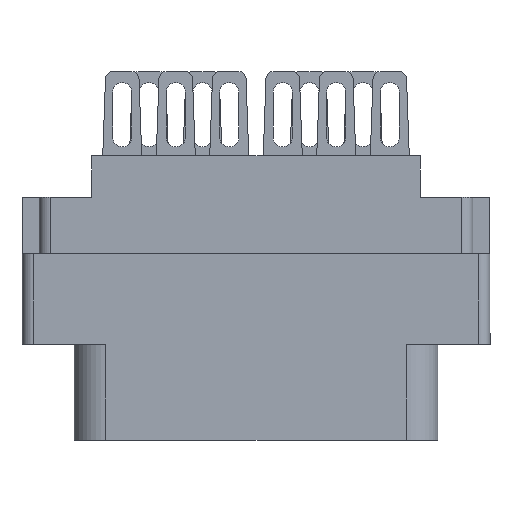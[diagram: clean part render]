
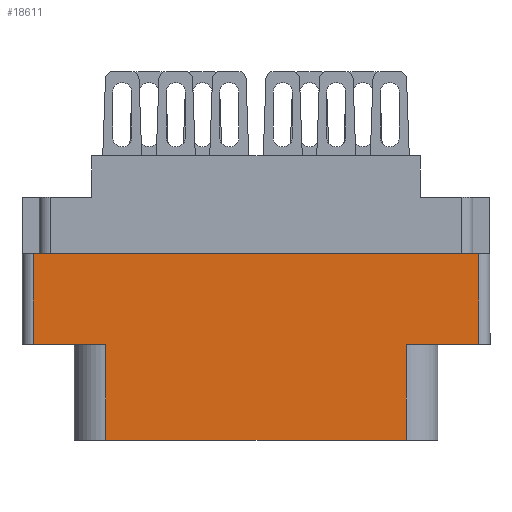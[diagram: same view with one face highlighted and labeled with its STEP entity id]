
A CAD part, front view. The second image highlights one B-rep face of the part: STEP entity #18611.
In plain terms, the highlighted planar face has unit normal (0, -1, 0).
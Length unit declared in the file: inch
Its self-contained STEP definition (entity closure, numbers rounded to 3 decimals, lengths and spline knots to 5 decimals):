
#87 = DIRECTION ( 'NONE',  ( 0., 0., 1. ) ) ;
#232 = VERTEX_POINT ( 'NONE', #1029 ) ;
#833 = LINE ( 'NONE', #1506, #4343 ) ;
#1029 = CARTESIAN_POINT ( 'NONE',  ( -0.42052, -0.343, -0.798 ) ) ;
#1467 = ORIENTED_EDGE ( 'NONE', *, *, #18213, .T. ) ;
#1506 = CARTESIAN_POINT ( 'NONE',  ( -0.624, -0.343, -0.798 ) ) ;
#1854 = ORIENTED_EDGE ( 'NONE', *, *, #9611, .F. ) ;
#2181 = EDGE_CURVE ( 'NONE', #17108, #22630, #7887, .T. ) ;
#2445 = CARTESIAN_POINT ( 'NONE',  ( -0.656, -0.343, -0.798 ) ) ;
#3041 = CARTESIAN_POINT ( 'NONE',  ( -0.624, -0.343, -0.529 ) ) ;
#3423 = CARTESIAN_POINT ( 'NONE',  ( -0.42052, -0.343, -0.529 ) ) ;
#4343 = VECTOR ( 'NONE', #18271, 39.37008 ) ;
#4677 = CARTESIAN_POINT ( 'NONE',  ( -0.42052, -0.343, -0.798 ) ) ;
#5013 = EDGE_CURVE ( 'NONE', #17108, #5492, #833, .T. ) ;
#5138 = CARTESIAN_POINT ( 'NONE',  ( 0.42052, -0.343, -0.529 ) ) ;
#5395 = CARTESIAN_POINT ( 'NONE',  ( 0., -0.343, -0.274 ) ) ;
#5452 = DIRECTION ( 'NONE',  ( 0., 0., 1. ) ) ;
#5492 = VERTEX_POINT ( 'NONE', #3041 ) ;
#5869 = CARTESIAN_POINT ( 'NONE',  ( 0.624, -0.343, -0.529 ) ) ;
#5897 = LINE ( 'NONE', #5138, #20418 ) ;
#6327 = ORIENTED_EDGE ( 'NONE', *, *, #17281, .T. ) ;
#7887 = LINE ( 'NONE', #5395, #17459 ) ;
#8630 = CARTESIAN_POINT ( 'NONE',  ( 0.624, -0.343, -0.274 ) ) ;
#8793 = DIRECTION ( 'NONE',  ( 0., 0., -1. ) ) ;
#9199 = ORIENTED_EDGE ( 'NONE', *, *, #20204, .T. ) ;
#9513 = VECTOR ( 'NONE', #87, 39.37008 ) ;
#9611 = EDGE_CURVE ( 'NONE', #13071, #13885, #12452, .T. ) ;
#10106 = LINE ( 'NONE', #22533, #9513 ) ;
#10127 = VECTOR ( 'NONE', #19437, 39.37008 ) ;
#10517 = VECTOR ( 'NONE', #22030, 39.37008 ) ;
#10795 = CARTESIAN_POINT ( 'NONE',  ( 0.42052, -0.343, -0.529 ) ) ;
#11306 = VERTEX_POINT ( 'NONE', #3423 ) ;
#12452 = LINE ( 'NONE', #13939, #20014 ) ;
#12926 = EDGE_CURVE ( 'NONE', #5492, #11306, #20375, .T. ) ;
#13071 = VERTEX_POINT ( 'NONE', #5869 ) ;
#13105 = ORIENTED_EDGE ( 'NONE', *, *, #2181, .F. ) ;
#13314 = ORIENTED_EDGE ( 'NONE', *, *, #21001, .T. ) ;
#13885 = VERTEX_POINT ( 'NONE', #10795 ) ;
#13939 = CARTESIAN_POINT ( 'NONE',  ( 0., -0.343, -0.529 ) ) ;
#14224 = CARTESIAN_POINT ( 'NONE',  ( 0., -0.343, -0.529 ) ) ;
#14421 = FACE_OUTER_BOUND ( 'NONE', #16275, .T. ) ;
#14530 = DIRECTION ( 'NONE',  ( 1., 0., 0. ) ) ;
#16069 = PLANE ( 'NONE',  #22063 ) ;
#16147 = CARTESIAN_POINT ( 'NONE',  ( -0.656, -0.343, -0.798 ) ) ;
#16275 = EDGE_LOOP ( 'NONE', ( #13105, #21007, #17529, #6327, #9199, #13314, #1854, #1467 ) ) ;
#16602 = CARTESIAN_POINT ( 'NONE',  ( 0.42052, -0.343, -0.798 ) ) ;
#16959 = VECTOR ( 'NONE', #20988, 39.37008 ) ;
#17108 = VERTEX_POINT ( 'NONE', #20423 ) ;
#17281 = EDGE_CURVE ( 'NONE', #11306, #232, #21148, .T. ) ;
#17459 = VECTOR ( 'NONE', #14530, 39.37008 ) ;
#17529 = ORIENTED_EDGE ( 'NONE', *, *, #12926, .T. ) ;
#18213 = EDGE_CURVE ( 'NONE', #13071, #22630, #10106, .T. ) ;
#18271 = DIRECTION ( 'NONE',  ( 0., 0., -1. ) ) ;
#18611 = ADVANCED_FACE ( 'NONE', ( #14421 ), #16069, .T. ) ;
#19437 = DIRECTION ( 'NONE',  ( 0., 0., -1. ) ) ;
#19486 = DIRECTION ( 'NONE',  ( -1., 0., 0. ) ) ;
#20014 = VECTOR ( 'NONE', #19486, 39.37008 ) ;
#20204 = EDGE_CURVE ( 'NONE', #232, #21746, #22207, .T. ) ;
#20375 = LINE ( 'NONE', #14224, #10517 ) ;
#20418 = VECTOR ( 'NONE', #5452, 39.37008 ) ;
#20423 = CARTESIAN_POINT ( 'NONE',  ( -0.624, -0.343, -0.274 ) ) ;
#20988 = DIRECTION ( 'NONE',  ( 1., 0., 0. ) ) ;
#21001 = EDGE_CURVE ( 'NONE', #21746, #13885, #5897, .T. ) ;
#21007 = ORIENTED_EDGE ( 'NONE', *, *, #5013, .T. ) ;
#21148 = LINE ( 'NONE', #4677, #10127 ) ;
#21746 = VERTEX_POINT ( 'NONE', #16602 ) ;
#21864 = DIRECTION ( 'NONE',  ( 0., -1., 0. ) ) ;
#22030 = DIRECTION ( 'NONE',  ( 1., 0., 0. ) ) ;
#22063 = AXIS2_PLACEMENT_3D ( 'NONE', #16147, #21864, #8793 ) ;
#22207 = LINE ( 'NONE', #2445, #16959 ) ;
#22533 = CARTESIAN_POINT ( 'NONE',  ( 0.624, -0.343, -0.798 ) ) ;
#22630 = VERTEX_POINT ( 'NONE', #8630 ) ;
